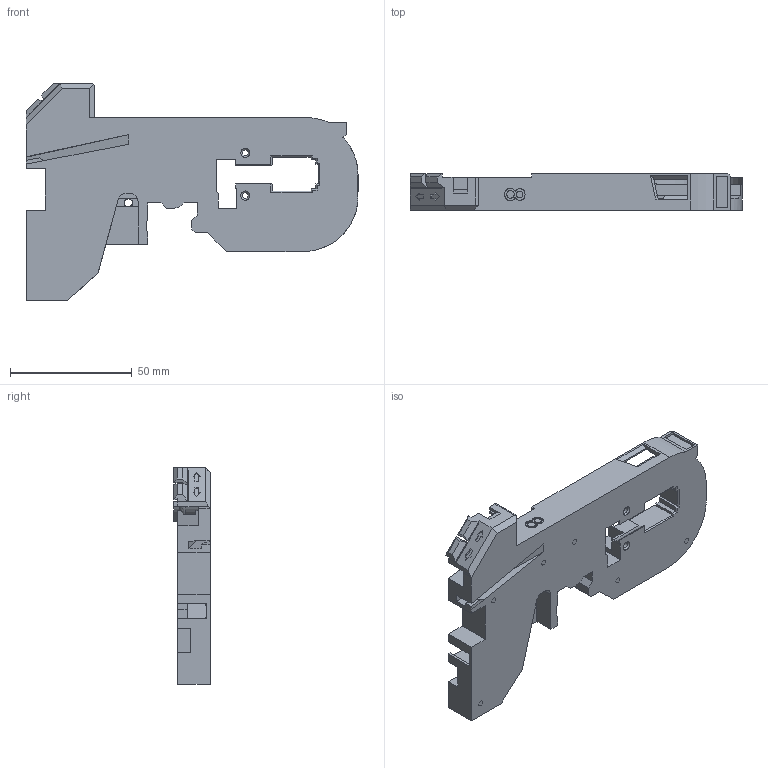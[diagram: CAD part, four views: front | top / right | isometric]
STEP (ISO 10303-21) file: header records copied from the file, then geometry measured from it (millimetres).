
FILE_DESCRIPTION(('FreeCAD Model'),'2;1');
FILE_NAME('Open CASCADE Shape Model','2025-01-14T15:10:23',(''),(''), 'Open CASCADE STEP processor 7.6','FreeCAD','Unknown');
FILE_SCHEMA(('AUTOMOTIVE_DESIGN { 1 0 10303 214 1 1 1 1 }'));
Length unit declared in the file: millimetre
Products named in the file (1): Compound
Bounding box: 136.25 x 15 x 88.9 mm (x, y, z)
Volume: 64155 mm3; surface area: 29937.9 mm2
Topology: 7 solids, 7 shells, 711 faces, 2225 edges, 1546 vertices
Faces by surface type: plane 391, bspline 204, extrusion 64, cylinder 39, cone 12, revolution 1
Full cylindrical faces by diameter (mm): 2.25 x7, 2.45 x2, 3.2 x1, 7 x1
Entity records: 34398 total; most frequent: CARTESIAN_POINT 10860, ORIENTED_EDGE 4446, DIRECTION 2928, EDGE_CURVE 2223, VERTEX_POINT 1546, VECTOR 1325, LINE 1261, AXIS2_PLACEMENT_3D 801
